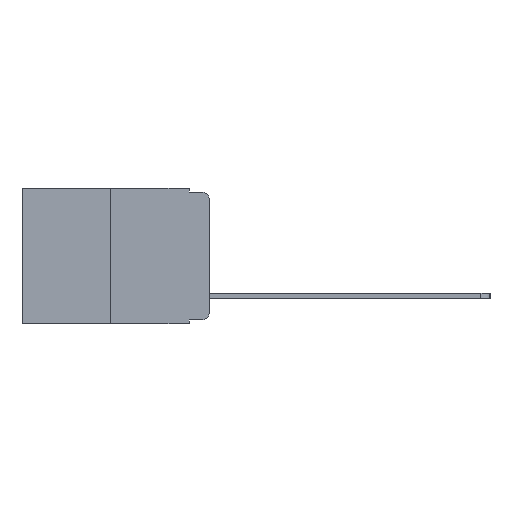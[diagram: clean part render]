
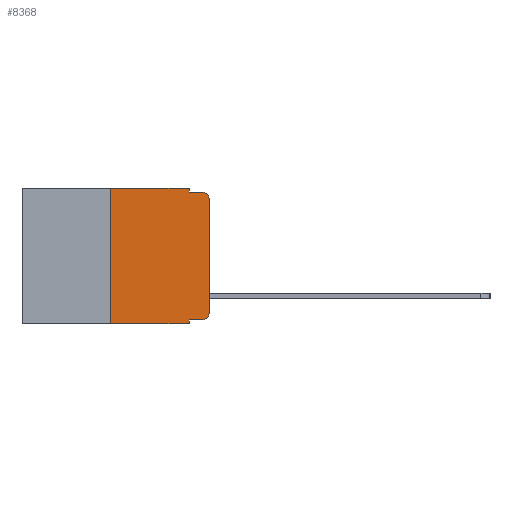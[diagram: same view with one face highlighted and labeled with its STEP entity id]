
A CAD part, left-side view. The second image highlights one B-rep face of the part: STEP entity #8368.
In plain terms, the highlighted planar face has unit normal (-1, 0, 0).
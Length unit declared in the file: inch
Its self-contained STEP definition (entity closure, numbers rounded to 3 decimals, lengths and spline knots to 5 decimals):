
#93 = ORIENTED_EDGE ( 'NONE', *, *, #960, .T. ) ;
#190 = ORIENTED_EDGE ( 'NONE', *, *, #651, .T. ) ;
#288 = DIRECTION ( 'NONE',  ( 0., 0., 1. ) ) ;
#329 = VERTEX_POINT ( 'NONE', #4303 ) ;
#426 = LINE ( 'NONE', #6632, #10708 ) ;
#620 = VECTOR ( 'NONE', #288, 39.37008 ) ;
#651 = EDGE_CURVE ( 'NONE', #10926, #6370, #7178, .T. ) ;
#869 = CARTESIAN_POINT ( 'NONE',  ( 0., 0., -0.03 ) ) ;
#960 = EDGE_CURVE ( 'NONE', #6370, #10513, #11114, .T. ) ;
#1330 = LINE ( 'NONE', #5594, #11383 ) ;
#1349 = LINE ( 'NONE', #4743, #11396 ) ;
#1426 = CARTESIAN_POINT ( 'NONE',  ( 0., 0.051, -0.343 ) ) ;
#1484 = DIRECTION ( 'NONE',  ( 0., 0., -1. ) ) ;
#1612 = CARTESIAN_POINT ( 'NONE',  ( 0., 0.02, -0.03 ) ) ;
#1728 = DIRECTION ( 'NONE',  ( 0., -1., 0. ) ) ;
#2366 = DIRECTION ( 'NONE',  ( 0., 0., -1. ) ) ;
#2529 = AXIS2_PLACEMENT_3D ( 'NONE', #1612, #8644, #2666 ) ;
#2666 = DIRECTION ( 'NONE',  ( 0., 0., -1. ) ) ;
#2699 = EDGE_CURVE ( 'NONE', #11656, #10926, #6838, .T. ) ;
#2904 = CARTESIAN_POINT ( 'NONE',  ( 0., 0.25, 0. ) ) ;
#3078 = LINE ( 'NONE', #2904, #10492 ) ;
#3251 = CARTESIAN_POINT ( 'NONE',  ( 0., 0., 0. ) ) ;
#3702 = CARTESIAN_POINT ( 'NONE',  ( 0., 0.02, -0.333 ) ) ;
#3739 = ORIENTED_EDGE ( 'NONE', *, *, #10842, .F. ) ;
#3949 = DIRECTION ( 'NONE',  ( 0., -1., 0. ) ) ;
#4201 = CARTESIAN_POINT ( 'NONE',  ( 0., 0.02, -0.313 ) ) ;
#4303 = CARTESIAN_POINT ( 'NONE',  ( 0., 0.051, -0.01 ) ) ;
#4682 = CARTESIAN_POINT ( 'NONE',  ( 0., 0.051, 0. ) ) ;
#4743 = CARTESIAN_POINT ( 'NONE',  ( 0., 0.051, 0. ) ) ;
#4797 = DIRECTION ( 'NONE',  ( -1., 0., 0. ) ) ;
#4835 = ORIENTED_EDGE ( 'NONE', *, *, #9276, .T. ) ;
#4918 = ORIENTED_EDGE ( 'NONE', *, *, #2699, .T. ) ;
#5064 = CARTESIAN_POINT ( 'NONE',  ( 0., 0.02, -0.01 ) ) ;
#5235 = EDGE_CURVE ( 'NONE', #11246, #7505, #7723, .T. ) ;
#5283 = PLANE ( 'NONE',  #9795 ) ;
#5594 = CARTESIAN_POINT ( 'NONE',  ( 0., 0.051, -0.01 ) ) ;
#5905 = CARTESIAN_POINT ( 'NONE',  ( 0., 0.473, 0. ) ) ;
#5966 = FACE_OUTER_BOUND ( 'NONE', #12096, .T. ) ;
#6321 = VERTEX_POINT ( 'NONE', #4682 ) ;
#6370 = VERTEX_POINT ( 'NONE', #11367 ) ;
#6379 = CIRCLE ( 'NONE', #2529, 0.02 ) ;
#6571 = DIRECTION ( 'NONE',  ( 0., -1., 0. ) ) ;
#6632 = CARTESIAN_POINT ( 'NONE',  ( 0., 0.051, 0. ) ) ;
#6838 = LINE ( 'NONE', #8683, #11373 ) ;
#6933 = DIRECTION ( 'NONE',  ( 0., -1., 0. ) ) ;
#7082 = LINE ( 'NONE', #5905, #11027 ) ;
#7178 = CIRCLE ( 'NONE', #11945, 0.02 ) ;
#7338 = DIRECTION ( 'NONE',  ( 0., 0., -1. ) ) ;
#7505 = VERTEX_POINT ( 'NONE', #1426 ) ;
#7723 = LINE ( 'NONE', #10743, #12173 ) ;
#7773 = EDGE_CURVE ( 'NONE', #11349, #6321, #7082, .T. ) ;
#7808 = ORIENTED_EDGE ( 'NONE', *, *, #9677, .F. ) ;
#7853 = EDGE_CURVE ( 'NONE', #11246, #11349, #3078, .T. ) ;
#8091 = ORIENTED_EDGE ( 'NONE', *, *, #7773, .F. ) ;
#8192 = CARTESIAN_POINT ( 'NONE',  ( 0., 0.25, -0.343 ) ) ;
#8368 = ADVANCED_FACE ( 'NONE', ( #5966 ), #5283, .F. ) ;
#8534 = ORIENTED_EDGE ( 'NONE', *, *, #5235, .T. ) ;
#8644 = DIRECTION ( 'NONE',  ( -1., 0., 0. ) ) ;
#8683 = CARTESIAN_POINT ( 'NONE',  ( 0., 0.051, -0.333 ) ) ;
#8924 = VERTEX_POINT ( 'NONE', #5064 ) ;
#9276 = EDGE_CURVE ( 'NONE', #10513, #8924, #6379, .T. ) ;
#9326 = ORIENTED_EDGE ( 'NONE', *, *, #10267, .F. ) ;
#9677 = EDGE_CURVE ( 'NONE', #6321, #329, #426, .T. ) ;
#9795 = AXIS2_PLACEMENT_3D ( 'NONE', #11798, #9987, #7338 ) ;
#9987 = DIRECTION ( 'NONE',  ( 1., 0., 0. ) ) ;
#10267 = EDGE_CURVE ( 'NONE', #11656, #7505, #1349, .T. ) ;
#10492 = VECTOR ( 'NONE', #12367, 39.37008 ) ;
#10513 = VERTEX_POINT ( 'NONE', #869 ) ;
#10708 = VECTOR ( 'NONE', #1484, 39.37008 ) ;
#10743 = CARTESIAN_POINT ( 'NONE',  ( 0., 0.473, -0.343 ) ) ;
#10842 = EDGE_CURVE ( 'NONE', #329, #8924, #1330, .T. ) ;
#10926 = VERTEX_POINT ( 'NONE', #3702 ) ;
#11027 = VECTOR ( 'NONE', #6933, 39.37008 ) ;
#11114 = LINE ( 'NONE', #3251, #620 ) ;
#11246 = VERTEX_POINT ( 'NONE', #8192 ) ;
#11306 = ORIENTED_EDGE ( 'NONE', *, *, #7853, .F. ) ;
#11330 = DIRECTION ( 'NONE',  ( 0., 0., -1. ) ) ;
#11349 = VERTEX_POINT ( 'NONE', #11908 ) ;
#11367 = CARTESIAN_POINT ( 'NONE',  ( 0., 0., -0.313 ) ) ;
#11373 = VECTOR ( 'NONE', #1728, 39.37008 ) ;
#11383 = VECTOR ( 'NONE', #6571, 39.37008 ) ;
#11396 = VECTOR ( 'NONE', #11330, 39.37008 ) ;
#11656 = VERTEX_POINT ( 'NONE', #12402 ) ;
#11798 = CARTESIAN_POINT ( 'NONE',  ( 0., 0.473, 0. ) ) ;
#11908 = CARTESIAN_POINT ( 'NONE',  ( 0., 0.25, 0. ) ) ;
#11945 = AXIS2_PLACEMENT_3D ( 'NONE', #4201, #4797, #2366 ) ;
#12096 = EDGE_LOOP ( 'NONE', ( #93, #4835, #3739, #7808, #8091, #11306, #8534, #9326, #4918, #190 ) ) ;
#12173 = VECTOR ( 'NONE', #3949, 39.37008 ) ;
#12367 = DIRECTION ( 'NONE',  ( 0., 0., 1. ) ) ;
#12402 = CARTESIAN_POINT ( 'NONE',  ( 0., 0.051, -0.333 ) ) ;
